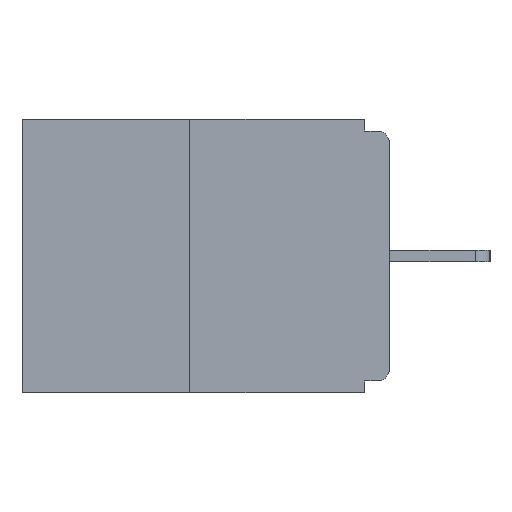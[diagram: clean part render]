
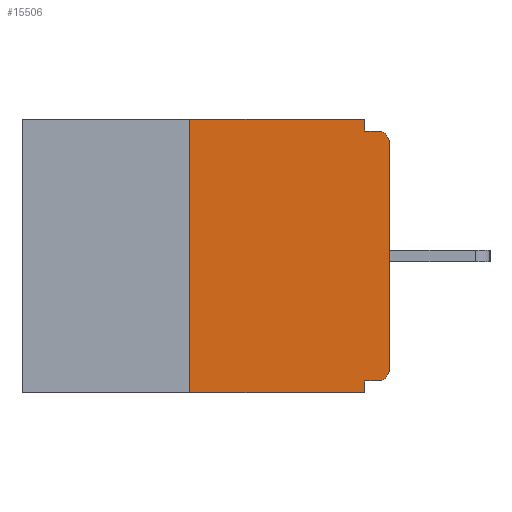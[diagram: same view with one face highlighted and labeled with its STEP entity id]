
A CAD part, left-side view. The second image highlights one B-rep face of the part: STEP entity #15506.
In plain terms, the highlighted planar face has unit normal (-1, 0, 0).
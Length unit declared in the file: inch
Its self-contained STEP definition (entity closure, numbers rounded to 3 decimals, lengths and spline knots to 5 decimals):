
#134 = LINE ( 'NONE', #1504, #10231 ) ;
#314 = AXIS2_PLACEMENT_3D ( 'NONE', #16960, #9373, #2666 ) ;
#863 = EDGE_CURVE ( 'NONE', #14485, #864, #5050, .T. ) ;
#864 = VERTEX_POINT ( 'NONE', #7690 ) ;
#869 = LINE ( 'NONE', #8876, #4321 ) ;
#1112 = DIRECTION ( 'NONE',  ( 0., 0., -1. ) ) ;
#1116 = DIRECTION ( 'NONE',  ( 0., -1., 0. ) ) ;
#1504 = CARTESIAN_POINT ( 'NONE',  ( 0., 0.46, 0. ) ) ;
#1957 = VECTOR ( 'NONE', #9552, 39.37008 ) ;
#2373 = CIRCLE ( 'NONE', #7031, 0.015 ) ;
#2469 = CARTESIAN_POINT ( 'NONE',  ( 0., 0.015, -0.328 ) ) ;
#2625 = EDGE_CURVE ( 'NONE', #864, #11653, #10686, .T. ) ;
#2666 = DIRECTION ( 'NONE',  ( 0., 0., -1. ) ) ;
#2677 = EDGE_CURVE ( 'NONE', #6170, #3900, #14993, .T. ) ;
#2692 = DIRECTION ( 'NONE',  ( 0., 0., -1. ) ) ;
#3149 = ORIENTED_EDGE ( 'NONE', *, *, #10105, .F. ) ;
#3474 = CARTESIAN_POINT ( 'NONE',  ( 0., 0.031, 0. ) ) ;
#3541 = EDGE_CURVE ( 'NONE', #6154, #7667, #5033, .T. ) ;
#3704 = DIRECTION ( 'NONE',  ( -1., 0., 0. ) ) ;
#3900 = VERTEX_POINT ( 'NONE', #13614 ) ;
#3914 = CARTESIAN_POINT ( 'NONE',  ( 0., 0.015, -0.313 ) ) ;
#4321 = VECTOR ( 'NONE', #14055, 39.37008 ) ;
#4398 = ORIENTED_EDGE ( 'NONE', *, *, #2677, .F. ) ;
#4707 = EDGE_CURVE ( 'NONE', #3900, #6154, #134, .T. ) ;
#4951 = CARTESIAN_POINT ( 'NONE',  ( 0., 0., -0.03 ) ) ;
#5033 = LINE ( 'NONE', #16723, #11525 ) ;
#5050 = CIRCLE ( 'NONE', #16842, 0.015 ) ;
#5092 = FACE_OUTER_BOUND ( 'NONE', #7891, .T. ) ;
#5394 = DIRECTION ( 'NONE',  ( 0., -1., 0. ) ) ;
#5449 = LINE ( 'NONE', #14597, #13247 ) ;
#5601 = DIRECTION ( 'NONE',  ( 0., 0., 1. ) ) ;
#6154 = VERTEX_POINT ( 'NONE', #3474 ) ;
#6170 = VERTEX_POINT ( 'NONE', #12710 ) ;
#6750 = DIRECTION ( 'NONE',  ( 0., 1., 0. ) ) ;
#7031 = AXIS2_PLACEMENT_3D ( 'NONE', #16703, #3704, #1112 ) ;
#7285 = LINE ( 'NONE', #16665, #10110 ) ;
#7667 = VERTEX_POINT ( 'NONE', #15641 ) ;
#7690 = CARTESIAN_POINT ( 'NONE',  ( 0., 0., -0.313 ) ) ;
#7743 = ORIENTED_EDGE ( 'NONE', *, *, #13161, .F. ) ;
#7826 = VERTEX_POINT ( 'NONE', #16135 ) ;
#7891 = EDGE_LOOP ( 'NONE', ( #8856, #4398, #9088, #3149, #7743, #15349, #8459, #15069, #12909, #10597 ) ) ;
#8276 = CARTESIAN_POINT ( 'NONE',  ( 0., 0.015, -0.015 ) ) ;
#8352 = CARTESIAN_POINT ( 'NONE',  ( 0., 0., 0. ) ) ;
#8359 = EDGE_CURVE ( 'NONE', #11653, #10294, #2373, .T. ) ;
#8459 = ORIENTED_EDGE ( 'NONE', *, *, #2625, .T. ) ;
#8856 = ORIENTED_EDGE ( 'NONE', *, *, #4707, .F. ) ;
#8876 = CARTESIAN_POINT ( 'NONE',  ( 0., 0.46, -0.343 ) ) ;
#9088 = ORIENTED_EDGE ( 'NONE', *, *, #9289, .T. ) ;
#9158 = DIRECTION ( 'NONE',  ( -1., 0., 0. ) ) ;
#9289 = EDGE_CURVE ( 'NONE', #6170, #9304, #869, .T. ) ;
#9304 = VERTEX_POINT ( 'NONE', #11285 ) ;
#9373 = DIRECTION ( 'NONE',  ( 1., 0., 0. ) ) ;
#9552 = DIRECTION ( 'NONE',  ( 0., 0., 1. ) ) ;
#9576 = VECTOR ( 'NONE', #5601, 39.37008 ) ;
#10105 = EDGE_CURVE ( 'NONE', #7826, #9304, #7285, .T. ) ;
#10110 = VECTOR ( 'NONE', #10128, 39.37008 ) ;
#10128 = DIRECTION ( 'NONE',  ( 0., 0., -1. ) ) ;
#10231 = VECTOR ( 'NONE', #5394, 39.37008 ) ;
#10294 = VERTEX_POINT ( 'NONE', #8276 ) ;
#10597 = ORIENTED_EDGE ( 'NONE', *, *, #3541, .F. ) ;
#10671 = CARTESIAN_POINT ( 'NONE',  ( 0., 0., -0.015 ) ) ;
#10686 = LINE ( 'NONE', #8352, #1957 ) ;
#11285 = CARTESIAN_POINT ( 'NONE',  ( 0., 0.031, -0.343 ) ) ;
#11525 = VECTOR ( 'NONE', #15182, 39.37008 ) ;
#11653 = VERTEX_POINT ( 'NONE', #4951 ) ;
#12710 = CARTESIAN_POINT ( 'NONE',  ( 0., 0.25, -0.343 ) ) ;
#12909 = ORIENTED_EDGE ( 'NONE', *, *, #15549, .F. ) ;
#13161 = EDGE_CURVE ( 'NONE', #14485, #7826, #5449, .T. ) ;
#13247 = VECTOR ( 'NONE', #6750, 39.37008 ) ;
#13611 = CARTESIAN_POINT ( 'NONE',  ( 0., 0.25, 0. ) ) ;
#13614 = CARTESIAN_POINT ( 'NONE',  ( 0., 0.25, 0. ) ) ;
#14055 = DIRECTION ( 'NONE',  ( 0., -1., 0. ) ) ;
#14485 = VERTEX_POINT ( 'NONE', #2469 ) ;
#14561 = PLANE ( 'NONE',  #314 ) ;
#14597 = CARTESIAN_POINT ( 'NONE',  ( 0., 0., -0.328 ) ) ;
#14644 = LINE ( 'NONE', #10671, #16273 ) ;
#14993 = LINE ( 'NONE', #13611, #9576 ) ;
#15069 = ORIENTED_EDGE ( 'NONE', *, *, #8359, .T. ) ;
#15182 = DIRECTION ( 'NONE',  ( 0., 0., -1. ) ) ;
#15349 = ORIENTED_EDGE ( 'NONE', *, *, #863, .T. ) ;
#15506 = ADVANCED_FACE ( 'NONE', ( #5092 ), #14561, .F. ) ;
#15549 = EDGE_CURVE ( 'NONE', #7667, #10294, #14644, .T. ) ;
#15641 = CARTESIAN_POINT ( 'NONE',  ( 0., 0.031, -0.015 ) ) ;
#16135 = CARTESIAN_POINT ( 'NONE',  ( 0., 0.031, -0.328 ) ) ;
#16273 = VECTOR ( 'NONE', #1116, 39.37008 ) ;
#16665 = CARTESIAN_POINT ( 'NONE',  ( 0., 0.031, -0.343 ) ) ;
#16703 = CARTESIAN_POINT ( 'NONE',  ( 0., 0.015, -0.03 ) ) ;
#16723 = CARTESIAN_POINT ( 'NONE',  ( 0., 0.031, 0. ) ) ;
#16842 = AXIS2_PLACEMENT_3D ( 'NONE', #3914, #9158, #2692 ) ;
#16960 = CARTESIAN_POINT ( 'NONE',  ( 0., 0.46, 0. ) ) ;
